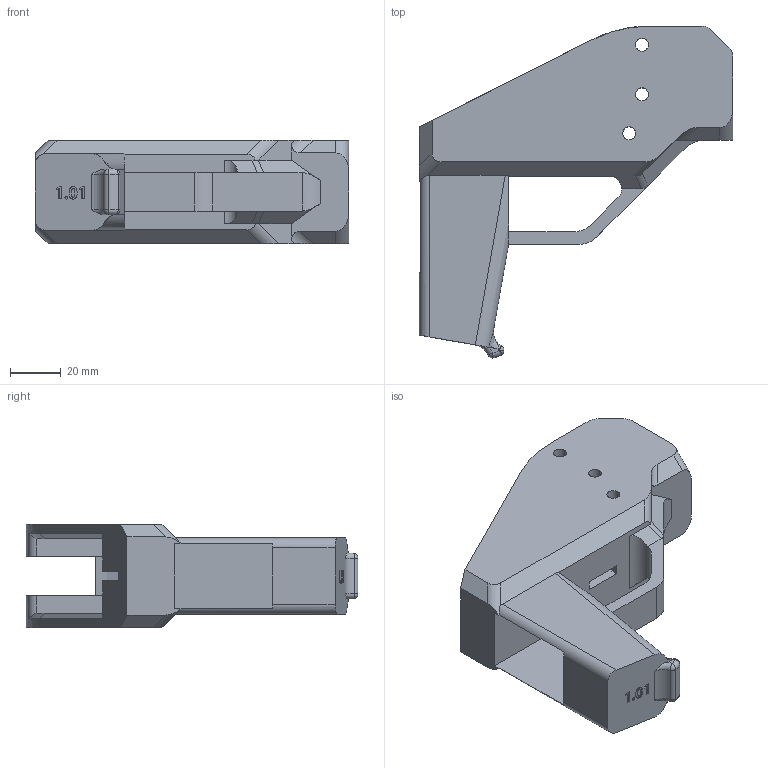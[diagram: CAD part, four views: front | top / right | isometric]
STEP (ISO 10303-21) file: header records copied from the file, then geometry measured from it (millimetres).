
FILE_DESCRIPTION (( 'STEP AP214' ), '1' );
FILE_NAME ('LiberatorCompact101.STEP', '2013-06-02T23:45:56', ( 'PVTCaboose1337' ), ( '' ), 'SwSTEP 2.0', 'SolidWorks 2013', '' );
FILE_SCHEMA (( 'AUTOMOTIVE_DESIGN' ));
Length unit declared in the file: millimetre
Products named in the file (1): LiberatorCompact101
Bounding box: 122.94 x 130.21 x 40.64 mm (x, y, z)
Volume: 147596.8 mm3; surface area: 47082.7 mm2
Topology: 1 solids, 1 shells, 206 faces, 581 edges, 379 vertices
Faces by surface type: plane 107, cylinder 57, bspline 18, torus 14, sphere 6, cone 4
Entity records: 7855 total; most frequent: CARTESIAN_POINT 2649, ORIENTED_EDGE 1154, DIRECTION 993, EDGE_CURVE 577, VERTEX_POINT 377, VECTOR 343, LINE 343, AXIS2_PLACEMENT_3D 325
